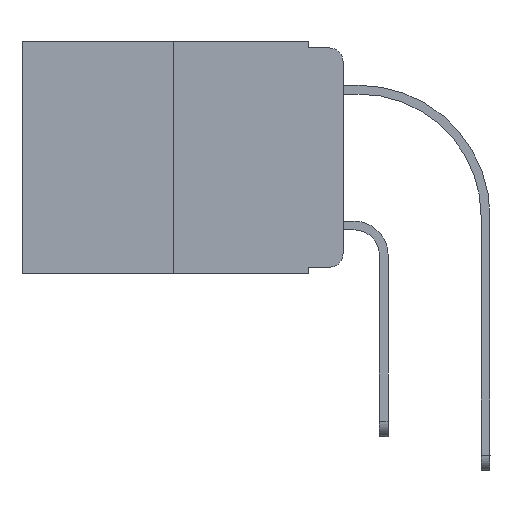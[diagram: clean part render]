
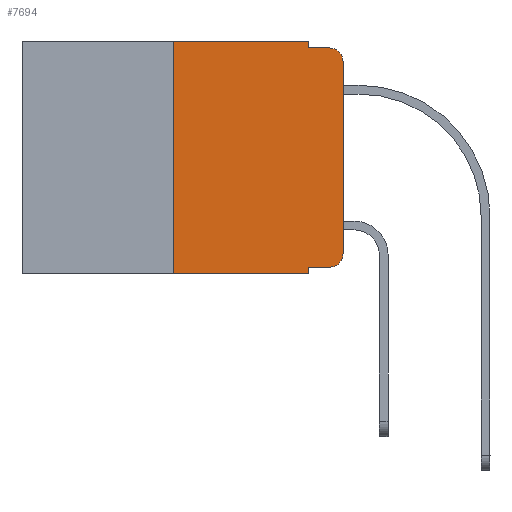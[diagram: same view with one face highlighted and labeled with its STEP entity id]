
A CAD part, left-side view. The second image highlights one B-rep face of the part: STEP entity #7694.
In plain terms, the highlighted planar face has unit normal (-1, 0, 0).
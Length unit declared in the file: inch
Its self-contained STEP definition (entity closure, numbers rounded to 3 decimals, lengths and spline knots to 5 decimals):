
#86 = DIRECTION ( 'NONE',  ( -1., 0., 0. ) ) ;
#289 = VERTEX_POINT ( 'NONE', #1891 ) ;
#301 = CARTESIAN_POINT ( 'NONE',  ( 0., 0.02, -0.03 ) ) ;
#600 = PLANE ( 'NONE',  #9660 ) ;
#780 = LINE ( 'NONE', #13785, #4309 ) ;
#865 = EDGE_CURVE ( 'NONE', #4227, #2372, #13188, .T. ) ;
#927 = ORIENTED_EDGE ( 'NONE', *, *, #8443, .T. ) ;
#1891 = CARTESIAN_POINT ( 'NONE',  ( 0., 0.25, 0. ) ) ;
#1928 = LINE ( 'NONE', #3273, #7929 ) ;
#2170 = DIRECTION ( 'NONE',  ( 0., -1., 0. ) ) ;
#2372 = VERTEX_POINT ( 'NONE', #15008 ) ;
#2446 = VECTOR ( 'NONE', #2170, 39.37008 ) ;
#2652 = DIRECTION ( 'NONE',  ( 0., 0., 1. ) ) ;
#2939 = CARTESIAN_POINT ( 'NONE',  ( 0., 0.25, 0. ) ) ;
#3273 = CARTESIAN_POINT ( 'NONE',  ( 0., 0.051, -0.01 ) ) ;
#3448 = ORIENTED_EDGE ( 'NONE', *, *, #10755, .F. ) ;
#3812 = LINE ( 'NONE', #10996, #8713 ) ;
#3883 = DIRECTION ( 'NONE',  ( 0., -1., 0. ) ) ;
#4080 = DIRECTION ( 'NONE',  ( -1., 0., 0. ) ) ;
#4203 = VECTOR ( 'NONE', #6845, 39.37008 ) ;
#4227 = VERTEX_POINT ( 'NONE', #12896 ) ;
#4251 = EDGE_CURVE ( 'NONE', #7718, #14409, #9370, .T. ) ;
#4309 = VECTOR ( 'NONE', #5496, 39.37008 ) ;
#4350 = AXIS2_PLACEMENT_3D ( 'NONE', #301, #4080, #5255 ) ;
#4892 = DIRECTION ( 'NONE',  ( 0., 0., -1. ) ) ;
#5163 = ORIENTED_EDGE ( 'NONE', *, *, #5625, .F. ) ;
#5255 = DIRECTION ( 'NONE',  ( 0., 0., -1. ) ) ;
#5291 = CARTESIAN_POINT ( 'NONE',  ( 0., 0.051, -0.343 ) ) ;
#5496 = DIRECTION ( 'NONE',  ( 0., -1., 0. ) ) ;
#5625 = EDGE_CURVE ( 'NONE', #9736, #8121, #3812, .T. ) ;
#5669 = EDGE_CURVE ( 'NONE', #289, #7718, #13429, .T. ) ;
#6148 = CARTESIAN_POINT ( 'NONE',  ( 0., 0.473, 0. ) ) ;
#6187 = LINE ( 'NONE', #13542, #12216 ) ;
#6739 = CARTESIAN_POINT ( 'NONE',  ( 0., 0.25, -0.343 ) ) ;
#6845 = DIRECTION ( 'NONE',  ( 0., 0., 1. ) ) ;
#6855 = ORIENTED_EDGE ( 'NONE', *, *, #4251, .F. ) ;
#6868 = VERTEX_POINT ( 'NONE', #6739 ) ;
#6972 = CARTESIAN_POINT ( 'NONE',  ( 0., 0.02, -0.01 ) ) ;
#7020 = CARTESIAN_POINT ( 'NONE',  ( 0., 0.473, -0.343 ) ) ;
#7460 = ORIENTED_EDGE ( 'NONE', *, *, #10762, .F. ) ;
#7694 = ADVANCED_FACE ( 'NONE', ( #7722 ), #600, .F. ) ;
#7718 = VERTEX_POINT ( 'NONE', #10621 ) ;
#7722 = FACE_OUTER_BOUND ( 'NONE', #13909, .T. ) ;
#7838 = CIRCLE ( 'NONE', #4350, 0.02 ) ;
#7929 = VECTOR ( 'NONE', #12808, 39.37008 ) ;
#8099 = ORIENTED_EDGE ( 'NONE', *, *, #11794, .T. ) ;
#8121 = VERTEX_POINT ( 'NONE', #5291 ) ;
#8443 = EDGE_CURVE ( 'NONE', #2372, #8521, #6187, .T. ) ;
#8521 = VERTEX_POINT ( 'NONE', #12683 ) ;
#8713 = VECTOR ( 'NONE', #14608, 39.37008 ) ;
#8982 = ORIENTED_EDGE ( 'NONE', *, *, #15395, .T. ) ;
#9164 = ORIENTED_EDGE ( 'NONE', *, *, #14092, .T. ) ;
#9370 = LINE ( 'NONE', #14163, #14449 ) ;
#9543 = CARTESIAN_POINT ( 'NONE',  ( 0., 0.051, -0.01 ) ) ;
#9582 = ORIENTED_EDGE ( 'NONE', *, *, #865, .T. ) ;
#9660 = AXIS2_PLACEMENT_3D ( 'NONE', #10147, #14930, #15016 ) ;
#9736 = VERTEX_POINT ( 'NONE', #12000 ) ;
#10147 = CARTESIAN_POINT ( 'NONE',  ( 0., 0.473, 0. ) ) ;
#10613 = CARTESIAN_POINT ( 'NONE',  ( 0., 0.02, -0.313 ) ) ;
#10621 = CARTESIAN_POINT ( 'NONE',  ( 0., 0.051, 0. ) ) ;
#10755 = EDGE_CURVE ( 'NONE', #6868, #289, #12648, .T. ) ;
#10762 = EDGE_CURVE ( 'NONE', #14409, #11100, #1928, .T. ) ;
#10996 = CARTESIAN_POINT ( 'NONE',  ( 0., 0.051, 0. ) ) ;
#11100 = VERTEX_POINT ( 'NONE', #6972 ) ;
#11477 = VECTOR ( 'NONE', #3883, 39.37008 ) ;
#11794 = EDGE_CURVE ( 'NONE', #6868, #8121, #12891, .T. ) ;
#11864 = ORIENTED_EDGE ( 'NONE', *, *, #5669, .F. ) ;
#12000 = CARTESIAN_POINT ( 'NONE',  ( 0., 0.051, -0.333 ) ) ;
#12216 = VECTOR ( 'NONE', #2652, 39.37008 ) ;
#12648 = LINE ( 'NONE', #2939, #4203 ) ;
#12683 = CARTESIAN_POINT ( 'NONE',  ( 0., 0., -0.03 ) ) ;
#12808 = DIRECTION ( 'NONE',  ( 0., -1., 0. ) ) ;
#12891 = LINE ( 'NONE', #7020, #2446 ) ;
#12896 = CARTESIAN_POINT ( 'NONE',  ( 0., 0.02, -0.333 ) ) ;
#12979 = DIRECTION ( 'NONE',  ( 0., 0., -1. ) ) ;
#13188 = CIRCLE ( 'NONE', #14443, 0.02 ) ;
#13429 = LINE ( 'NONE', #6148, #11477 ) ;
#13542 = CARTESIAN_POINT ( 'NONE',  ( 0., 0., 0. ) ) ;
#13785 = CARTESIAN_POINT ( 'NONE',  ( 0., 0.051, -0.333 ) ) ;
#13909 = EDGE_LOOP ( 'NONE', ( #927, #9164, #7460, #6855, #11864, #3448, #8099, #5163, #8982, #9582 ) ) ;
#14092 = EDGE_CURVE ( 'NONE', #8521, #11100, #7838, .T. ) ;
#14163 = CARTESIAN_POINT ( 'NONE',  ( 0., 0.051, 0. ) ) ;
#14409 = VERTEX_POINT ( 'NONE', #9543 ) ;
#14443 = AXIS2_PLACEMENT_3D ( 'NONE', #10613, #86, #4892 ) ;
#14449 = VECTOR ( 'NONE', #12979, 39.37008 ) ;
#14608 = DIRECTION ( 'NONE',  ( 0., 0., -1. ) ) ;
#14930 = DIRECTION ( 'NONE',  ( 1., 0., 0. ) ) ;
#15008 = CARTESIAN_POINT ( 'NONE',  ( 0., 0., -0.313 ) ) ;
#15016 = DIRECTION ( 'NONE',  ( 0., 0., -1. ) ) ;
#15395 = EDGE_CURVE ( 'NONE', #9736, #4227, #780, .T. ) ;
